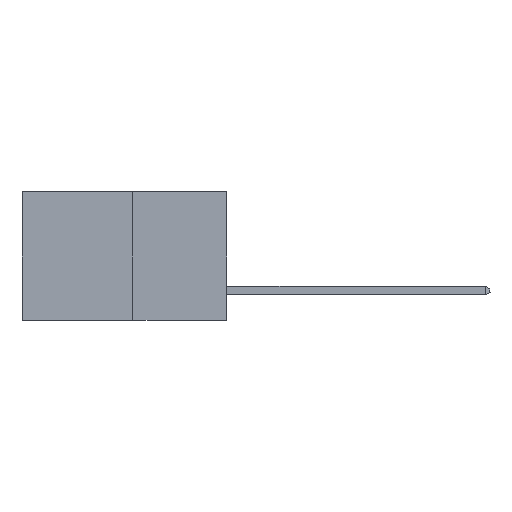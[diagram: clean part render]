
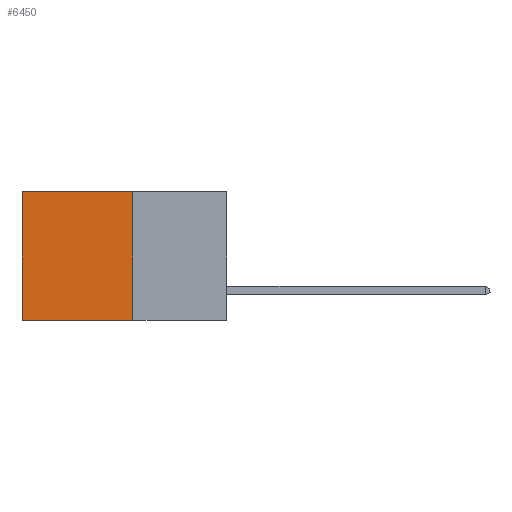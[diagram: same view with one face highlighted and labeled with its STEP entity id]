
A CAD part, left-side view. The second image highlights one B-rep face of the part: STEP entity #6450.
In plain terms, the highlighted planar face has unit normal (-1, 0, 0).
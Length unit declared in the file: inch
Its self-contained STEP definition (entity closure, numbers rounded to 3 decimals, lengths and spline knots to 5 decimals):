
#469 = LINE ( 'NONE', #2589, #16120 ) ;
#913 = CARTESIAN_POINT ( 'NONE',  ( 0.277, 0.27, -0.37 ) ) ;
#1637 = FACE_OUTER_BOUND ( 'NONE', #3624, .T. ) ;
#1664 = LINE ( 'NONE', #19407, #2352 ) ;
#2352 = VECTOR ( 'NONE', #8876, 39.37008 ) ;
#2559 = DIRECTION ( 'NONE',  ( 0., 1., 0. ) ) ;
#2589 = CARTESIAN_POINT ( 'NONE',  ( 0.277, 0.27, -0.37 ) ) ;
#3380 = ORIENTED_EDGE ( 'NONE', *, *, #17102, .T. ) ;
#3624 = EDGE_LOOP ( 'NONE', ( #18876, #13502, #17938, #3380 ) ) ;
#5032 = CARTESIAN_POINT ( 'NONE',  ( 0.277, 0.59, -0.37 ) ) ;
#6450 = ADVANCED_FACE ( 'NONE', ( #1637 ), #10550, .F. ) ;
#6766 = CARTESIAN_POINT ( 'NONE',  ( 0.277, 0.59, 0. ) ) ;
#8328 = LINE ( 'NONE', #16610, #24502 ) ;
#8577 = VERTEX_POINT ( 'NONE', #6766 ) ;
#8876 = DIRECTION ( 'NONE',  ( 0., 0., -1. ) ) ;
#10455 = DIRECTION ( 'NONE',  ( 0., 0., -1. ) ) ;
#10478 = DIRECTION ( 'NONE',  ( 1., 0., 0. ) ) ;
#10550 = PLANE ( 'NONE',  #15473 ) ;
#10606 = CARTESIAN_POINT ( 'NONE',  ( 0.277, 0.27, -0.37 ) ) ;
#10739 = EDGE_CURVE ( 'NONE', #10878, #14500, #469, .T. ) ;
#10878 = VERTEX_POINT ( 'NONE', #913 ) ;
#11254 = CARTESIAN_POINT ( 'NONE',  ( 0.277, 0.27, 0. ) ) ;
#11962 = VECTOR ( 'NONE', #13378, 39.37008 ) ;
#13378 = DIRECTION ( 'NONE',  ( 0., 1., 0. ) ) ;
#13502 = ORIENTED_EDGE ( 'NONE', *, *, #10739, .F. ) ;
#14500 = VERTEX_POINT ( 'NONE', #5032 ) ;
#15473 = AXIS2_PLACEMENT_3D ( 'NONE', #10606, #10478, #10455 ) ;
#16120 = VECTOR ( 'NONE', #2559, 39.37008 ) ;
#16610 = CARTESIAN_POINT ( 'NONE',  ( 0.277, 0.27, -0.37 ) ) ;
#17102 = EDGE_CURVE ( 'NONE', #23689, #8577, #17617, .T. ) ;
#17440 = EDGE_CURVE ( 'NONE', #23689, #10878, #8328, .T. ) ;
#17617 = LINE ( 'NONE', #11254, #11962 ) ;
#17938 = ORIENTED_EDGE ( 'NONE', *, *, #17440, .F. ) ;
#18876 = ORIENTED_EDGE ( 'NONE', *, *, #22854, .T. ) ;
#19407 = CARTESIAN_POINT ( 'NONE',  ( 0.277, 0.59, -0.37 ) ) ;
#19935 = CARTESIAN_POINT ( 'NONE',  ( 0.277, 0.27, 0. ) ) ;
#22854 = EDGE_CURVE ( 'NONE', #8577, #14500, #1664, .T. ) ;
#23689 = VERTEX_POINT ( 'NONE', #19935 ) ;
#24502 = VECTOR ( 'NONE', #24973, 39.37008 ) ;
#24973 = DIRECTION ( 'NONE',  ( 0., 0., -1. ) ) ;
